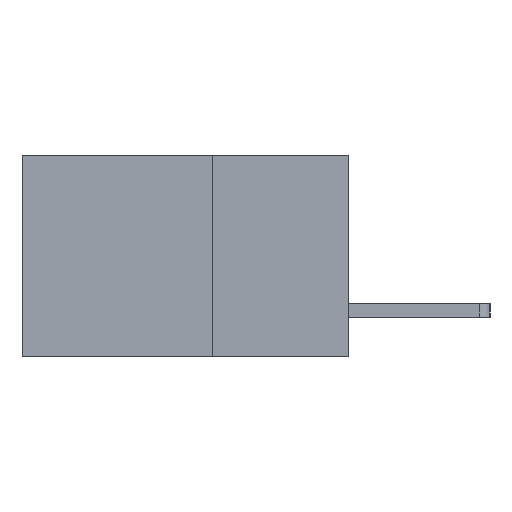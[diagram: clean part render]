
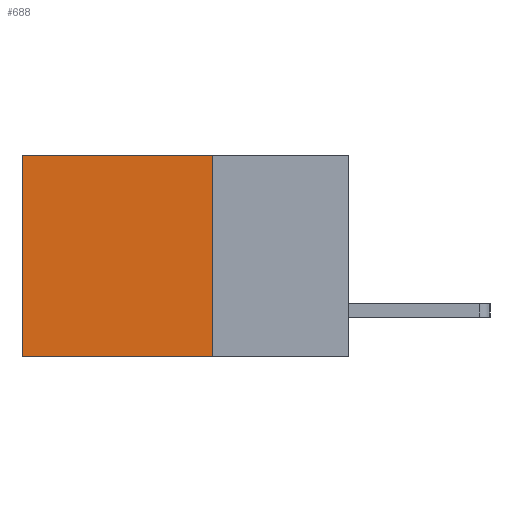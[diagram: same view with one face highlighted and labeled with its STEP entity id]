
A CAD part, left-side view. The second image highlights one B-rep face of the part: STEP entity #688.
In plain terms, the highlighted planar face has unit normal (-1, 0, 0).
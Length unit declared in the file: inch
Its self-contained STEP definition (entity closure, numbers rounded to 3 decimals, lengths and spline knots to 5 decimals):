
#337 = CARTESIAN_POINT ( 'NONE',  ( 0.2615, 0.6, -0.37 ) ) ;
#482 = VECTOR ( 'NONE', #6150, 39.37008 ) ;
#568 = CARTESIAN_POINT ( 'NONE',  ( 0.2615, 0.25, -0.37 ) ) ;
#688 = ADVANCED_FACE ( 'NONE', ( #1629 ), #3990, .F. ) ;
#814 = LINE ( 'NONE', #568, #2097 ) ;
#992 = CARTESIAN_POINT ( 'NONE',  ( 0.2615, 0.6, 0. ) ) ;
#1206 = CARTESIAN_POINT ( 'NONE',  ( 0.2615, 0.25, -0.37 ) ) ;
#1308 = DIRECTION ( 'NONE',  ( 0., 0., -1. ) ) ;
#1327 = VECTOR ( 'NONE', #1308, 39.37008 ) ;
#1576 = LINE ( 'NONE', #2870, #8158 ) ;
#1614 = ORIENTED_EDGE ( 'NONE', *, *, #4017, .F. ) ;
#1629 = FACE_OUTER_BOUND ( 'NONE', #6793, .T. ) ;
#1867 = VERTEX_POINT ( 'NONE', #337 ) ;
#2097 = VECTOR ( 'NONE', #5047, 39.37008 ) ;
#2572 = CARTESIAN_POINT ( 'NONE',  ( 0.2615, 0.6, -0.37 ) ) ;
#2870 = CARTESIAN_POINT ( 'NONE',  ( 0.2615, 0.25, 0. ) ) ;
#3058 = ORIENTED_EDGE ( 'NONE', *, *, #7888, .T. ) ;
#3439 = ORIENTED_EDGE ( 'NONE', *, *, #6802, .F. ) ;
#3929 = VERTEX_POINT ( 'NONE', #992 ) ;
#3990 = PLANE ( 'NONE',  #5210 ) ;
#4017 = EDGE_CURVE ( 'NONE', #4689, #1867, #5568, .T. ) ;
#4689 = VERTEX_POINT ( 'NONE', #1206 ) ;
#5035 = VERTEX_POINT ( 'NONE', #6652 ) ;
#5047 = DIRECTION ( 'NONE',  ( 0., 0., -1. ) ) ;
#5210 = AXIS2_PLACEMENT_3D ( 'NONE', #7132, #7282, #5752 ) ;
#5568 = LINE ( 'NONE', #6822, #482 ) ;
#5605 = EDGE_CURVE ( 'NONE', #3929, #1867, #8110, .T. ) ;
#5752 = DIRECTION ( 'NONE',  ( 0., 0., -1. ) ) ;
#6150 = DIRECTION ( 'NONE',  ( 0., 1., 0. ) ) ;
#6652 = CARTESIAN_POINT ( 'NONE',  ( 0.2615, 0.25, 0. ) ) ;
#6776 = ORIENTED_EDGE ( 'NONE', *, *, #5605, .T. ) ;
#6793 = EDGE_LOOP ( 'NONE', ( #6776, #1614, #3439, #3058 ) ) ;
#6802 = EDGE_CURVE ( 'NONE', #5035, #4689, #814, .T. ) ;
#6822 = CARTESIAN_POINT ( 'NONE',  ( 0.2615, 0.25, -0.37 ) ) ;
#7132 = CARTESIAN_POINT ( 'NONE',  ( 0.2615, 0.25, -0.37 ) ) ;
#7282 = DIRECTION ( 'NONE',  ( 1., 0., 0. ) ) ;
#7888 = EDGE_CURVE ( 'NONE', #5035, #3929, #1576, .T. ) ;
#7987 = DIRECTION ( 'NONE',  ( 0., 1., 0. ) ) ;
#8110 = LINE ( 'NONE', #2572, #1327 ) ;
#8158 = VECTOR ( 'NONE', #7987, 39.37008 ) ;
